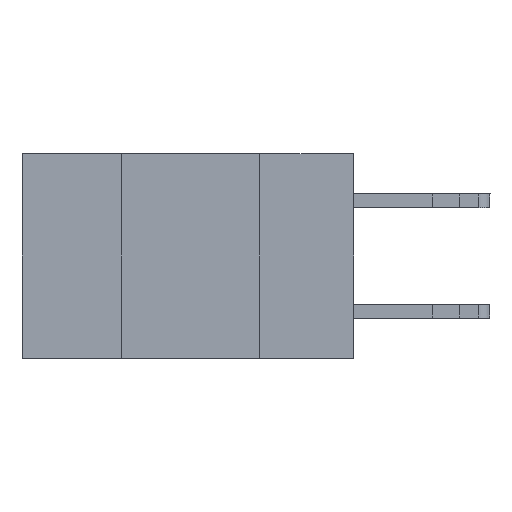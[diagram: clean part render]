
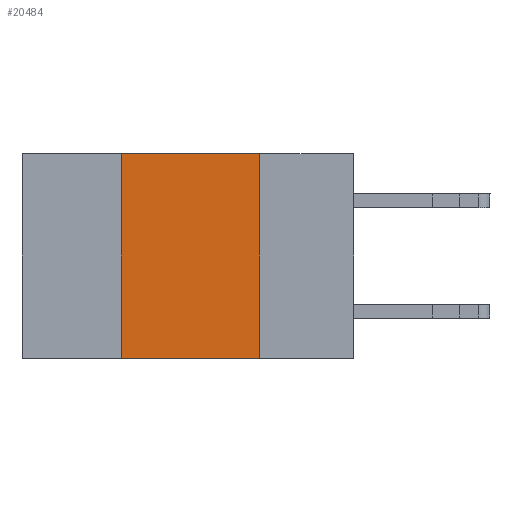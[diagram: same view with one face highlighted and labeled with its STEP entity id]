
A CAD part, left-side view. The second image highlights one B-rep face of the part: STEP entity #20484.
In plain terms, the highlighted planar face has unit normal (-1, 0, 0).
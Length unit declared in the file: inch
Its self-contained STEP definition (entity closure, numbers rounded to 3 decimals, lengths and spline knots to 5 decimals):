
#1946 = PLANE ( 'NONE',  #16247 ) ;
#2013 = DIRECTION ( 'NONE',  ( 1., 0., 0. ) ) ;
#2181 = CARTESIAN_POINT ( 'NONE',  ( 0., 0.17, 0. ) ) ;
#3598 = EDGE_CURVE ( 'NONE', #15352, #3676, #13292, .T. ) ;
#3676 = VERTEX_POINT ( 'NONE', #19258 ) ;
#3903 = DIRECTION ( 'NONE',  ( 0., 0., -1. ) ) ;
#4470 = ORIENTED_EDGE ( 'NONE', *, *, #13201, .F. ) ;
#4623 = VERTEX_POINT ( 'NONE', #21628 ) ;
#5099 = DIRECTION ( 'NONE',  ( 0., -1., 0. ) ) ;
#7304 = CARTESIAN_POINT ( 'NONE',  ( 0., 0.42, 0. ) ) ;
#7651 = VECTOR ( 'NONE', #5099, 39.37008 ) ;
#8812 = FACE_OUTER_BOUND ( 'NONE', #18956, .T. ) ;
#10060 = VECTOR ( 'NONE', #17636, 39.37008 ) ;
#10401 = VECTOR ( 'NONE', #20291, 39.37008 ) ;
#11608 = CARTESIAN_POINT ( 'NONE',  ( 0., 0.17, 0. ) ) ;
#12506 = LINE ( 'NONE', #7304, #13859 ) ;
#12790 = DIRECTION ( 'NONE',  ( 0., 0., 1. ) ) ;
#13201 = EDGE_CURVE ( 'NONE', #15352, #4623, #12506, .T. ) ;
#13292 = LINE ( 'NONE', #19412, #10060 ) ;
#13859 = VECTOR ( 'NONE', #12790, 39.37008 ) ;
#15352 = VERTEX_POINT ( 'NONE', #16095 ) ;
#16065 = ORIENTED_EDGE ( 'NONE', *, *, #21918, .F. ) ;
#16095 = CARTESIAN_POINT ( 'NONE',  ( 0., 0.42, -0.37 ) ) ;
#16247 = AXIS2_PLACEMENT_3D ( 'NONE', #19271, #2013, #3903 ) ;
#16319 = EDGE_CURVE ( 'NONE', #4623, #22406, #19074, .T. ) ;
#17636 = DIRECTION ( 'NONE',  ( 0., -1., 0. ) ) ;
#18687 = CARTESIAN_POINT ( 'NONE',  ( 0., 0.6, 0. ) ) ;
#18708 = ORIENTED_EDGE ( 'NONE', *, *, #3598, .T. ) ;
#18956 = EDGE_LOOP ( 'NONE', ( #16065, #20237, #4470, #18708 ) ) ;
#19074 = LINE ( 'NONE', #18687, #7651 ) ;
#19258 = CARTESIAN_POINT ( 'NONE',  ( 0., 0.17, -0.37 ) ) ;
#19271 = CARTESIAN_POINT ( 'NONE',  ( 0., 0.6, 0. ) ) ;
#19412 = CARTESIAN_POINT ( 'NONE',  ( 0., 0.6, -0.37 ) ) ;
#19940 = LINE ( 'NONE', #11608, #10401 ) ;
#20237 = ORIENTED_EDGE ( 'NONE', *, *, #16319, .F. ) ;
#20291 = DIRECTION ( 'NONE',  ( 0., 0., -1. ) ) ;
#20484 = ADVANCED_FACE ( 'NONE', ( #8812 ), #1946, .F. ) ;
#21628 = CARTESIAN_POINT ( 'NONE',  ( 0., 0.42, 0. ) ) ;
#21918 = EDGE_CURVE ( 'NONE', #22406, #3676, #19940, .T. ) ;
#22406 = VERTEX_POINT ( 'NONE', #2181 ) ;
